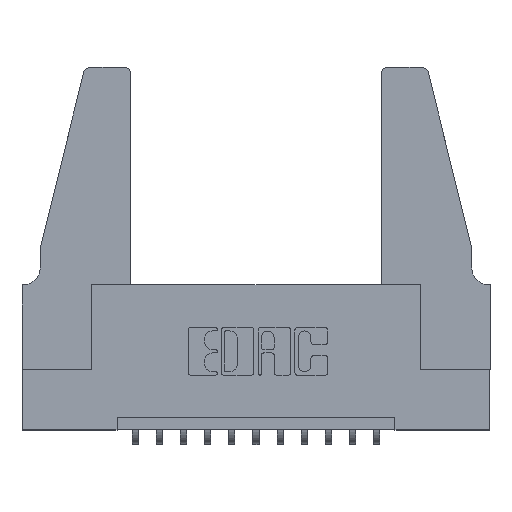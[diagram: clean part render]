
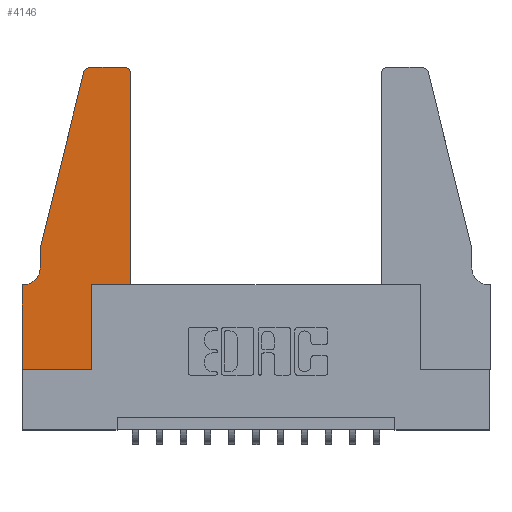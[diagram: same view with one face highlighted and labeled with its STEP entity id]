
A CAD part, top view. The second image highlights one B-rep face of the part: STEP entity #4146.
In plain terms, the highlighted planar face has unit normal (0, 0, 1).
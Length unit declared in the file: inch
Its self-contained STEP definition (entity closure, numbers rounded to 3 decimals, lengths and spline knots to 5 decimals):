
#52 = VERTEX_POINT ( 'NONE', #11212 ) ;
#99 = VECTOR ( 'NONE', #5855, 39.37008 ) ;
#101 = CARTESIAN_POINT ( 'NONE',  ( 0.0755, 0.35, 0.37 ) ) ;
#152 = LINE ( 'NONE', #3264, #7424 ) ;
#247 = CARTESIAN_POINT ( 'NONE',  ( 0., 0., 0.37 ) ) ;
#298 = CARTESIAN_POINT ( 'NONE',  ( 0., 0.35, 0.37 ) ) ;
#375 = EDGE_CURVE ( 'NONE', #8306, #4234, #3801, .T. ) ;
#384 = LINE ( 'NONE', #14037, #8875 ) ;
#444 = EDGE_CURVE ( 'NONE', #52, #12275, #11274, .T. ) ;
#595 = DIRECTION ( 'NONE',  ( -1., 0., 0. ) ) ;
#640 = EDGE_CURVE ( 'NONE', #11322, #1148, #3092, .T. ) ;
#787 = VECTOR ( 'NONE', #8128, 39.37008 ) ;
#990 = DIRECTION ( 'NONE',  ( 0., 1., 0. ) ) ;
#1148 = VERTEX_POINT ( 'NONE', #298 ) ;
#1323 = CARTESIAN_POINT ( 'NONE',  ( 0.4505, 0.35, 0.37 ) ) ;
#1397 = DIRECTION ( 'NONE',  ( 0., 0., -1. ) ) ;
#1409 = CARTESIAN_POINT ( 'NONE',  ( 0.0755, 0.5, 0.37 ) ) ;
#1460 = CARTESIAN_POINT ( 'NONE',  ( 0., 0., 0.37 ) ) ;
#1519 = CARTESIAN_POINT ( 'NONE',  ( 0.2865, 0., 0.37 ) ) ;
#1602 = ORIENTED_EDGE ( 'NONE', *, *, #2854, .T. ) ;
#1796 = FACE_OUTER_BOUND ( 'NONE', #3914, .T. ) ;
#2344 = DIRECTION ( 'NONE',  ( 1., 0., 0. ) ) ;
#2535 = CARTESIAN_POINT ( 'NONE',  ( 0.0055, 0.42, 0.37 ) ) ;
#2801 = EDGE_CURVE ( 'NONE', #5314, #52, #384, .T. ) ;
#2854 = EDGE_CURVE ( 'NONE', #1148, #3704, #9053, .T. ) ;
#2890 = ORIENTED_EDGE ( 'NONE', *, *, #6186, .T. ) ;
#2969 = ORIENTED_EDGE ( 'NONE', *, *, #8652, .T. ) ;
#2978 = ORIENTED_EDGE ( 'NONE', *, *, #3555, .T. ) ;
#3051 = VECTOR ( 'NONE', #10526, 39.37008 ) ;
#3092 = LINE ( 'NONE', #101, #787 ) ;
#3253 = LINE ( 'NONE', #1323, #14108 ) ;
#3264 = CARTESIAN_POINT ( 'NONE',  ( 0.2865, 0.35, 0.37 ) ) ;
#3397 = LINE ( 'NONE', #1409, #3051 ) ;
#3404 = CARTESIAN_POINT ( 'NONE',  ( 0.2865, 0.35, 0.37 ) ) ;
#3555 = EDGE_CURVE ( 'NONE', #13930, #6750, #152, .T. ) ;
#3611 = LINE ( 'NONE', #7221, #6979 ) ;
#3704 = VERTEX_POINT ( 'NONE', #247 ) ;
#3801 = LINE ( 'NONE', #4341, #14111 ) ;
#3908 = ORIENTED_EDGE ( 'NONE', *, *, #13685, .T. ) ;
#3914 = EDGE_LOOP ( 'NONE', ( #9974, #2969, #5061, #11797, #3908, #8014, #1602, #2890, #2978, #9684, #8444, #14579 ) ) ;
#4062 = CARTESIAN_POINT ( 'NONE',  ( 0.4505, 0.35, 0.37 ) ) ;
#4146 = ADVANCED_FACE ( 'NONE', ( #1796 ), #7015, .T. ) ;
#4234 = VERTEX_POINT ( 'NONE', #11871 ) ;
#4341 = CARTESIAN_POINT ( 'NONE',  ( 0.0755, 0.5, 0.37 ) ) ;
#5046 = DIRECTION ( 'NONE',  ( 1., 0., 0. ) ) ;
#5061 = ORIENTED_EDGE ( 'NONE', *, *, #375, .T. ) ;
#5224 = CARTESIAN_POINT ( 'NONE',  ( 0.25487, 1.22718, 0.37 ) ) ;
#5282 = VECTOR ( 'NONE', #14087, 39.37008 ) ;
#5314 = VERTEX_POINT ( 'NONE', #4062 ) ;
#5666 = DIRECTION ( 'NONE',  ( 1., 0., 0. ) ) ;
#5855 = DIRECTION ( 'NONE',  ( 1., 0., 0. ) ) ;
#6186 = EDGE_CURVE ( 'NONE', #3704, #13930, #12350, .T. ) ;
#6585 = CIRCLE ( 'NONE', #9147, 0.03 ) ;
#6750 = VERTEX_POINT ( 'NONE', #3404 ) ;
#6952 = DIRECTION ( 'NONE',  ( 1., 0., 0. ) ) ;
#6979 = VECTOR ( 'NONE', #595, 39.37008 ) ;
#7015 = PLANE ( 'NONE',  #10561 ) ;
#7136 = EDGE_CURVE ( 'NONE', #12275, #12141, #3611, .T. ) ;
#7221 = CARTESIAN_POINT ( 'NONE',  ( 0.2605, 1.25, 0.37 ) ) ;
#7424 = VECTOR ( 'NONE', #990, 39.37008 ) ;
#7917 = CARTESIAN_POINT ( 'NONE',  ( 0.4205, 1.22, 0.37 ) ) ;
#8014 = ORIENTED_EDGE ( 'NONE', *, *, #640, .T. ) ;
#8128 = DIRECTION ( 'NONE',  ( -1., 0., 0. ) ) ;
#8306 = VERTEX_POINT ( 'NONE', #5224 ) ;
#8444 = ORIENTED_EDGE ( 'NONE', *, *, #2801, .T. ) ;
#8652 = EDGE_CURVE ( 'NONE', #12141, #8306, #6585, .T. ) ;
#8812 = CARTESIAN_POINT ( 'NONE',  ( 0.0055, 0.35, 0.37 ) ) ;
#8875 = VECTOR ( 'NONE', #12818, 39.37008 ) ;
#8974 = EDGE_CURVE ( 'NONE', #4234, #14711, #3397, .T. ) ;
#9053 = LINE ( 'NONE', #1460, #5282 ) ;
#9147 = AXIS2_PLACEMENT_3D ( 'NONE', #10837, #10647, #5046 ) ;
#9251 = DIRECTION ( 'NONE',  ( 0., 0., 1. ) ) ;
#9684 = ORIENTED_EDGE ( 'NONE', *, *, #13253, .T. ) ;
#9974 = ORIENTED_EDGE ( 'NONE', *, *, #7136, .T. ) ;
#10421 = CARTESIAN_POINT ( 'NONE',  ( 0., 0., 0.37 ) ) ;
#10526 = DIRECTION ( 'NONE',  ( 0., -1., 0. ) ) ;
#10561 = AXIS2_PLACEMENT_3D ( 'NONE', #13862, #9251, #6952 ) ;
#10647 = DIRECTION ( 'NONE',  ( 0., 0., 1. ) ) ;
#10837 = CARTESIAN_POINT ( 'NONE',  ( 0.284, 1.22, 0.37 ) ) ;
#11119 = DIRECTION ( 'NONE',  ( -0.239, -0.971, 0. ) ) ;
#11212 = CARTESIAN_POINT ( 'NONE',  ( 0.4505, 1.22, 0.37 ) ) ;
#11274 = CIRCLE ( 'NONE', #13533, 0.03 ) ;
#11322 = VERTEX_POINT ( 'NONE', #8812 ) ;
#11671 = CARTESIAN_POINT ( 'NONE',  ( 0.284, 1.25, 0.37 ) ) ;
#11797 = ORIENTED_EDGE ( 'NONE', *, *, #8974, .T. ) ;
#11871 = CARTESIAN_POINT ( 'NONE',  ( 0.0755, 0.5, 0.37 ) ) ;
#12141 = VERTEX_POINT ( 'NONE', #11671 ) ;
#12169 = AXIS2_PLACEMENT_3D ( 'NONE', #2535, #1397, #12811 ) ;
#12275 = VERTEX_POINT ( 'NONE', #13841 ) ;
#12350 = LINE ( 'NONE', #10421, #99 ) ;
#12811 = DIRECTION ( 'NONE',  ( -1., 0., 0. ) ) ;
#12818 = DIRECTION ( 'NONE',  ( 0., 1., 0. ) ) ;
#13253 = EDGE_CURVE ( 'NONE', #6750, #5314, #3253, .T. ) ;
#13404 = CIRCLE ( 'NONE', #12169, 0.07 ) ;
#13533 = AXIS2_PLACEMENT_3D ( 'NONE', #7917, #13547, #2344 ) ;
#13547 = DIRECTION ( 'NONE',  ( 0., 0., 1. ) ) ;
#13685 = EDGE_CURVE ( 'NONE', #14711, #11322, #13404, .T. ) ;
#13841 = CARTESIAN_POINT ( 'NONE',  ( 0.4205, 1.25, 0.37 ) ) ;
#13862 = CARTESIAN_POINT ( 'NONE',  ( 0., 0.35, 0.37 ) ) ;
#13930 = VERTEX_POINT ( 'NONE', #1519 ) ;
#14012 = CARTESIAN_POINT ( 'NONE',  ( 0.0755, 0.42, 0.37 ) ) ;
#14037 = CARTESIAN_POINT ( 'NONE',  ( 0.4505, 0.35, 0.37 ) ) ;
#14087 = DIRECTION ( 'NONE',  ( 0., -1., 0. ) ) ;
#14108 = VECTOR ( 'NONE', #5666, 39.37008 ) ;
#14111 = VECTOR ( 'NONE', #11119, 39.37008 ) ;
#14579 = ORIENTED_EDGE ( 'NONE', *, *, #444, .T. ) ;
#14711 = VERTEX_POINT ( 'NONE', #14012 ) ;
